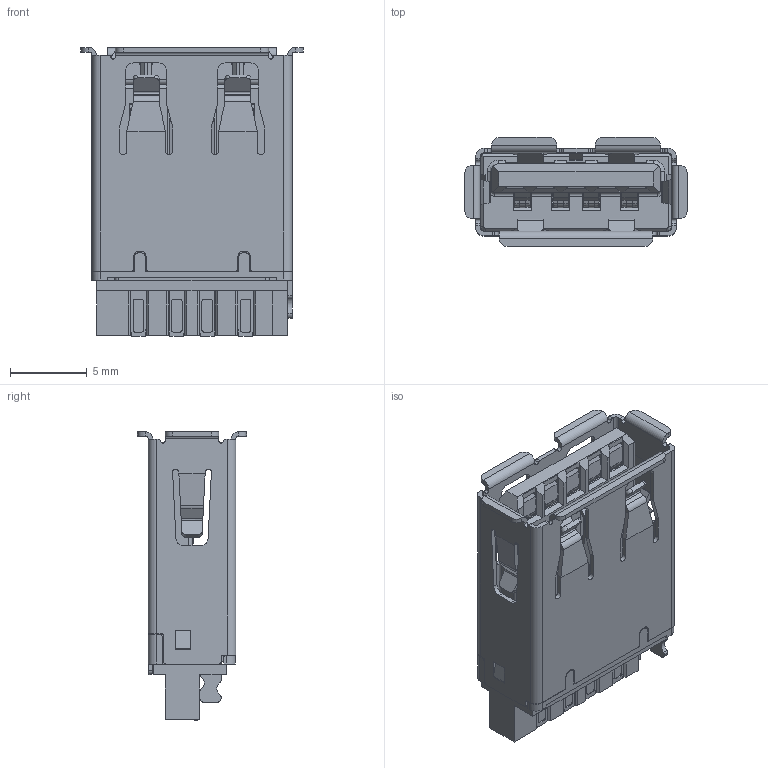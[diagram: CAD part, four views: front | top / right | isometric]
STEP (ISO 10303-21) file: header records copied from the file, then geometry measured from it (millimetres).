
FILE_DESCRIPTION (( 'STEP AP214' ), '1' );
FILE_NAME ('690M109-1AD-022.STEP', '2021-01-14T18:51:50', ( '' ), ( '' ), 'SwSTEP 2.0', 'SolidWorks 2020', '' );
FILE_SCHEMA (( 'AUTOMOTIVE_DESIGN' ));
Length unit declared in the file: millimetre
Products named in the file (9): Contact5 3.0 690M109-XAD-02X; Contact4 690M109-XAD-02X; Contact2 690M109-XAD-02X; Insulator1 690M109-XAD-02X_Blue; Contact3 690M109-XAD-02X; Contact1 690M109-XAD-02X; Insulator2 690M109-XAD-02X_Blue; 690M109-1AD-022; Shell 690M109-XAD-02X
Assembly tree (12 placements, depth 2):
  690M109-1AD-022
    Insulator1 690M109-XAD-02X_Blue
    Shell 690M109-XAD-02X
    Contact5 3.0 690M109-XAD-02X  x5
    Contact1 690M109-XAD-02X
    Contact2 690M109-XAD-02X
    Contact3 690M109-XAD-02X
    Contact4 690M109-XAD-02X
    Insulator2 690M109-XAD-02X_Blue
Bounding box: 14.5 x 7.12 x 18.86 mm (x, y, z)
Volume: 632 mm3; surface area: 2767.4 mm2
Topology: 12 solids, 12 shells, 2114 faces, 6047 edges, 3929 vertices
Faces by surface type: plane 1344, cylinder 654, bspline 114, cone 2
Entity records: 57174 total; most frequent: CARTESIAN_POINT 11776, ORIENTED_EDGE 9822, DIRECTION 9017, EDGE_CURVE 4911, VECTOR 3777, LINE 3777, VERTEX_POINT 3193, AXIS2_PLACEMENT_3D 2620
